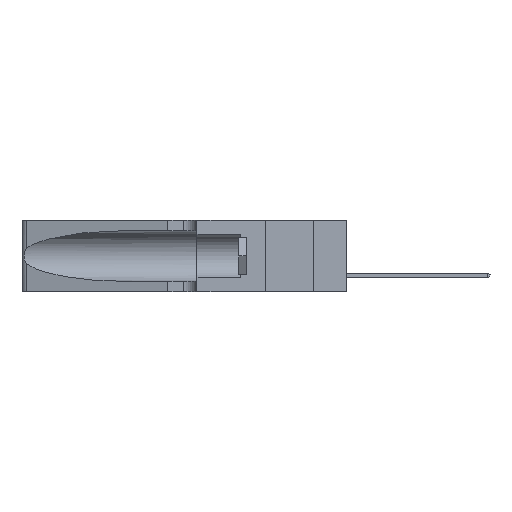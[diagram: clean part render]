
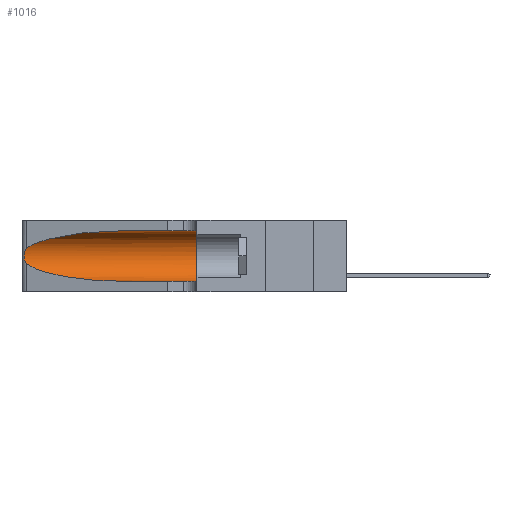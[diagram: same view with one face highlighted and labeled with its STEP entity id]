
A CAD part, left-side view. The second image highlights one B-rep face of the part: STEP entity #1016.
In plain terms, the highlighted cylindrical face has radius 3.308 mm (diameter 6.617 mm), a partial arc.
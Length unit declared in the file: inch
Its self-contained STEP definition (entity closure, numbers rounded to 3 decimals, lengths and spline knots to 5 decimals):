
#81 = CARTESIAN_POINT ( 'NONE',  ( 0.1305, 0.35, 0.185 ) ) ;
#157 = CARTESIAN_POINT ( 'NONE',  ( 0.2373, 1.15595, 0.28018 ) ) ;
#186 = ORIENTED_EDGE ( 'NONE', *, *, #44253, .T. ) ;
#842 = VECTOR ( 'NONE', #4801, 39.37008 ) ;
#1016 = ADVANCED_FACE ( 'NONE', ( #21647 ), #3051, .F. ) ;
#1111 = CARTESIAN_POINT ( 'NONE',  ( 0.1305, 1.61858, 0.31525 ) ) ;
#2304 = EDGE_CURVE ( 'NONE', #9018, #33069, #26837, .T. ) ;
#3051 = CYLINDRICAL_SURFACE ( 'NONE', #7173, 0.13025 ) ;
#3312 = CARTESIAN_POINT ( 'NONE',  ( 0.25856, 1.23593, 0.16098 ) ) ;
#3579 = CARTESIAN_POINT ( 'NONE',  ( 0.25487, 1.22718, 0.22369 ) ) ;
#3781 = EDGE_CURVE ( 'NONE', #41085, #33069, #35475, .T. ) ;
#4801 = DIRECTION ( 'NONE',  ( 0., -1., 0. ) ) ;
#5752 = B_SPLINE_CURVE_WITH_KNOTS ( 'NONE', 3,
 ( #3579, #24206, #24340, #20659, #6535, #41974, #13452, #38172, #17092, #3312, #14023, #28166, #10067, #20507 ),
 .UNSPECIFIED., .F., .F.,
 ( 4, 2, 2, 2, 2, 2, 4 ),
 ( 0., 0.00027, 0.00053, 0.00107, 0.0016, 0.00187, 0.00214 ),
 .UNSPECIFIED. ) ;
#6535 = CARTESIAN_POINT ( 'NONE',  ( 0.25854, 1.2359, 0.20912 ) ) ;
#7173 = AXIS2_PLACEMENT_3D ( 'NONE', #39302, #28443, #32005 ) ;
#9018 = VERTEX_POINT ( 'NONE', #33043 ) ;
#10067 = CARTESIAN_POINT ( 'NONE',  ( 0.25555, 1.22993, 0.14849 ) ) ;
#11272 = CARTESIAN_POINT ( 'NONE',  ( 0.1305, 0.72297, 0.31525 ) ) ;
#11493 = VERTEX_POINT ( 'NONE', #27292 ) ;
#11852 = ORIENTED_EDGE ( 'NONE', *, *, #2304, .F. ) ;
#13102 = CARTESIAN_POINT ( 'NONE',  ( 0.1305, 0.72297, 0.05475 ) ) ;
#13452 = CARTESIAN_POINT ( 'NONE',  ( 0.26075, 1.23896, 0.19203 ) ) ;
#13548 = CARTESIAN_POINT ( 'NONE',  ( 0.25487, 1.22718, 0.14631 ) ) ;
#14023 = CARTESIAN_POINT ( 'NONE',  ( 0.25789, 1.23486, 0.15765 ) ) ;
#14024 = LINE ( 'NONE', #1111, #842 ) ;
#15999 = VERTEX_POINT ( 'NONE', #39263 ) ;
#16222 = ORIENTED_EDGE ( 'NONE', *, *, #38475, .T. ) ;
#16457 = CARTESIAN_POINT ( 'NONE',  ( 0.18966, 0.96281, 0.05475 ) ) ;
#17092 = CARTESIAN_POINT ( 'NONE',  ( 0.26017, 1.23833, 0.17102 ) ) ;
#17258 =( BOUNDED_CURVE ( )  B_SPLINE_CURVE ( 3, ( #34059, #37834, #16457, #45034 ),
 .UNSPECIFIED., .F., .F. ) 
 B_SPLINE_CURVE_WITH_KNOTS ( ( 4, 4 ),
 ( 3.44316, 4.71239 ),
 .UNSPECIFIED. ) 
 CURVE ( )  GEOMETRIC_REPRESENTATION_ITEM ( )  RATIONAL_B_SPLINE_CURVE ( ( 1., 0.87, 0.87, 1. ) ) 
 REPRESENTATION_ITEM ( '' )  );
#18086 = DIRECTION ( 'NONE',  ( 0., -1., 0. ) ) ;
#18518 = ORIENTED_EDGE ( 'NONE', *, *, #25294, .F. ) ;
#20507 = CARTESIAN_POINT ( 'NONE',  ( 0.25487, 1.22718, 0.14631 ) ) ;
#20659 = CARTESIAN_POINT ( 'NONE',  ( 0.25787, 1.23484, 0.2124 ) ) ;
#21647 = FACE_OUTER_BOUND ( 'NONE', #37790, .T. ) ;
#22495 = AXIS2_PLACEMENT_3D ( 'NONE', #81, #27561, #28278 ) ;
#22808 = VECTOR ( 'NONE', #18086, 39.37008 ) ;
#22810 = CARTESIAN_POINT ( 'NONE',  ( 0.1305, 0.35, 0.05475 ) ) ;
#23185 = VERTEX_POINT ( 'NONE', #13548 ) ;
#24206 = CARTESIAN_POINT ( 'NONE',  ( 0.25555, 1.22994, 0.2215 ) ) ;
#24340 = CARTESIAN_POINT ( 'NONE',  ( 0.25639, 1.23184, 0.21858 ) ) ;
#25294 = EDGE_CURVE ( 'NONE', #15999, #9018, #14024, .T. ) ;
#26837 = CIRCLE ( 'NONE', #22495, 0.13025 ) ;
#27292 = CARTESIAN_POINT ( 'NONE',  ( 0.25487, 1.22718, 0.22369 ) ) ;
#27561 = DIRECTION ( 'NONE',  ( 0., 1., 0. ) ) ;
#28166 = CARTESIAN_POINT ( 'NONE',  ( 0.25639, 1.23186, 0.15144 ) ) ;
#28278 = DIRECTION ( 'NONE',  ( 0., 0., 1. ) ) ;
#28443 = DIRECTION ( 'NONE',  ( 0., -1., 0. ) ) ;
#28518 = CARTESIAN_POINT ( 'NONE',  ( 0.18966, 0.96281, 0.31525 ) ) ;
#31813 = CARTESIAN_POINT ( 'NONE',  ( 0.25487, 1.22718, 0.22369 ) ) ;
#32005 = DIRECTION ( 'NONE',  ( 0., 0., -1. ) ) ;
#32105 = ORIENTED_EDGE ( 'NONE', *, *, #3781, .T. ) ;
#33043 = CARTESIAN_POINT ( 'NONE',  ( 0.1305, 0.35, 0.31525 ) ) ;
#33069 = VERTEX_POINT ( 'NONE', #22810 ) ;
#33106 =( BOUNDED_CURVE ( )  B_SPLINE_CURVE ( 3, ( #11272, #28518, #157, #31813 ),
 .UNSPECIFIED., .F., .T. ) 
 B_SPLINE_CURVE_WITH_KNOTS ( ( 4, 4 ),
 ( 1.5708, 2.84003 ),
 .UNSPECIFIED. ) 
 CURVE ( )  GEOMETRIC_REPRESENTATION_ITEM ( )  RATIONAL_B_SPLINE_CURVE ( ( 1., 0.87, 0.87, 1. ) ) 
 REPRESENTATION_ITEM ( '' )  );
#34059 = CARTESIAN_POINT ( 'NONE',  ( 0.25487, 1.22718, 0.14631 ) ) ;
#35475 = LINE ( 'NONE', #37240, #22808 ) ;
#37240 = CARTESIAN_POINT ( 'NONE',  ( 0.1305, 1.61858, 0.05475 ) ) ;
#37790 = EDGE_LOOP ( 'NONE', ( #16222, #186, #38095, #32105, #11852, #18518 ) ) ;
#37834 = CARTESIAN_POINT ( 'NONE',  ( 0.2373, 1.15595, 0.08982 ) ) ;
#38095 = ORIENTED_EDGE ( 'NONE', *, *, #41086, .T. ) ;
#38172 = CARTESIAN_POINT ( 'NONE',  ( 0.26075, 1.23896, 0.178 ) ) ;
#38475 = EDGE_CURVE ( 'NONE', #15999, #11493, #33106, .T. ) ;
#39263 = CARTESIAN_POINT ( 'NONE',  ( 0.1305, 0.72297, 0.31525 ) ) ;
#39302 = CARTESIAN_POINT ( 'NONE',  ( 0.1305, 1.61858, 0.185 ) ) ;
#41085 = VERTEX_POINT ( 'NONE', #13102 ) ;
#41086 = EDGE_CURVE ( 'NONE', #23185, #41085, #17258, .T. ) ;
#41974 = CARTESIAN_POINT ( 'NONE',  ( 0.26018, 1.23835, 0.19895 ) ) ;
#44253 = EDGE_CURVE ( 'NONE', #11493, #23185, #5752, .T. ) ;
#45034 = CARTESIAN_POINT ( 'NONE',  ( 0.1305, 0.72297, 0.05475 ) ) ;
